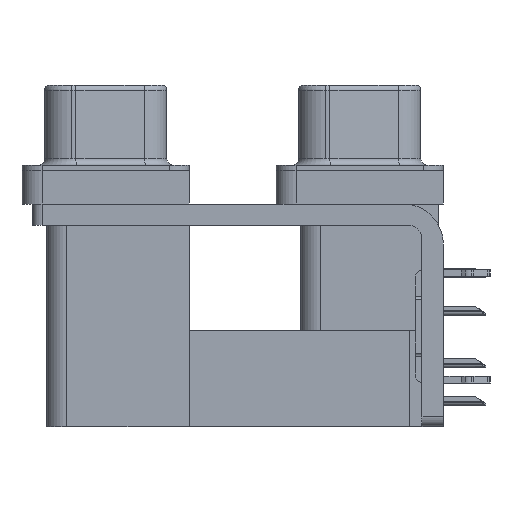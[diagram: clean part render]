
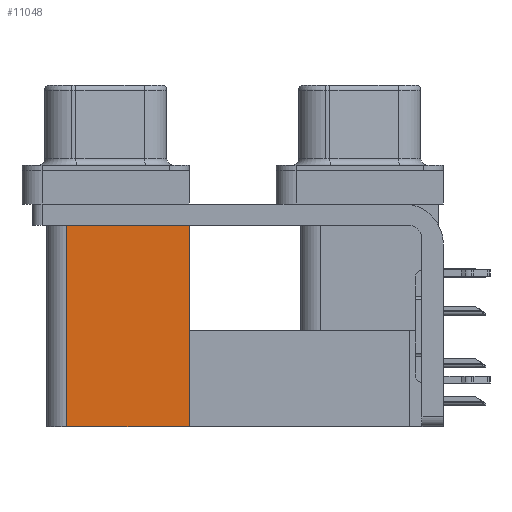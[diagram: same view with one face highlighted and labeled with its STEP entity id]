
A CAD part, left-side view. The second image highlights one B-rep face of the part: STEP entity #11048.
In plain terms, the highlighted planar face has unit normal (-1, 0, 0).
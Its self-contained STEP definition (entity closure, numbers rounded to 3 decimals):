
#819 = CARTESIAN_POINT ( 'NONE',  ( 3.7, 21.975, -19.2 ) ) ;
#999 = LINE ( 'NONE', #20548, #13173 ) ;
#2223 = EDGE_LOOP ( 'NONE', ( #34170, #3105, #17726, #12120 ) ) ;
#2555 = VERTEX_POINT ( 'NONE', #23086 ) ;
#3105 = ORIENTED_EDGE ( 'NONE', *, *, #22484, .F. ) ;
#4241 = DIRECTION ( 'NONE',  ( 1., 0., 0. ) ) ;
#6663 = PLANE ( 'NONE',  #11778 ) ;
#7585 = DIRECTION ( 'NONE',  ( 0., 1., 0. ) ) ;
#7807 = CARTESIAN_POINT ( 'NONE',  ( 3.7, 12.775, -2.5 ) ) ;
#8569 = EDGE_CURVE ( 'NONE', #36896, #13923, #27769, .T. ) ;
#8653 = CARTESIAN_POINT ( 'NONE',  ( 3.7, 21.975, -2.5 ) ) ;
#11041 = EDGE_CURVE ( 'NONE', #21821, #36896, #999, .T. ) ;
#11048 = ADVANCED_FACE ( 'NONE', ( #40716 ), #6663, .F. ) ;
#11778 = AXIS2_PLACEMENT_3D ( 'NONE', #20761, #4241, #27493 ) ;
#12120 = ORIENTED_EDGE ( 'NONE', *, *, #11041, .T. ) ;
#12752 = EDGE_CURVE ( 'NONE', #21821, #2555, #29624, .T. ) ;
#13173 = VECTOR ( 'NONE', #14281, 1000. ) ;
#13923 = VERTEX_POINT ( 'NONE', #8653 ) ;
#14281 = DIRECTION ( 'NONE',  ( 0., 0., 1. ) ) ;
#17726 = ORIENTED_EDGE ( 'NONE', *, *, #12752, .F. ) ;
#20548 = CARTESIAN_POINT ( 'NONE',  ( 3.7, 12.775, -19.2 ) ) ;
#20761 = CARTESIAN_POINT ( 'NONE',  ( 3.7, 12.775, -19.2 ) ) ;
#21821 = VERTEX_POINT ( 'NONE', #27662 ) ;
#22484 = EDGE_CURVE ( 'NONE', #2555, #13923, #29704, .T. ) ;
#23086 = CARTESIAN_POINT ( 'NONE',  ( 3.7, 21.975, -19.2 ) ) ;
#24091 = VECTOR ( 'NONE', #7585, 1000. ) ;
#24903 = CARTESIAN_POINT ( 'NONE',  ( 3.7, 12.775, -19.2 ) ) ;
#27493 = DIRECTION ( 'NONE',  ( 0., 1., 0. ) ) ;
#27662 = CARTESIAN_POINT ( 'NONE',  ( 3.7, 12.775, -19.2 ) ) ;
#27769 = LINE ( 'NONE', #7807, #24091 ) ;
#29624 = LINE ( 'NONE', #24903, #37409 ) ;
#29704 = LINE ( 'NONE', #819, #34097 ) ;
#33112 = CARTESIAN_POINT ( 'NONE',  ( 3.7, 12.775, -2.5 ) ) ;
#34097 = VECTOR ( 'NONE', #41167, 1000. ) ;
#34170 = ORIENTED_EDGE ( 'NONE', *, *, #8569, .T. ) ;
#36896 = VERTEX_POINT ( 'NONE', #33112 ) ;
#37409 = VECTOR ( 'NONE', #42850, 1000. ) ;
#40716 = FACE_OUTER_BOUND ( 'NONE', #2223, .T. ) ;
#41167 = DIRECTION ( 'NONE',  ( 0., 0., 1. ) ) ;
#42850 = DIRECTION ( 'NONE',  ( 0., 1., 0. ) ) ;
